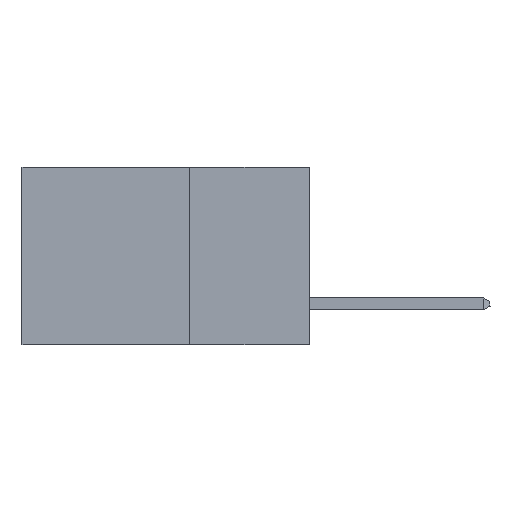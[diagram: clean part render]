
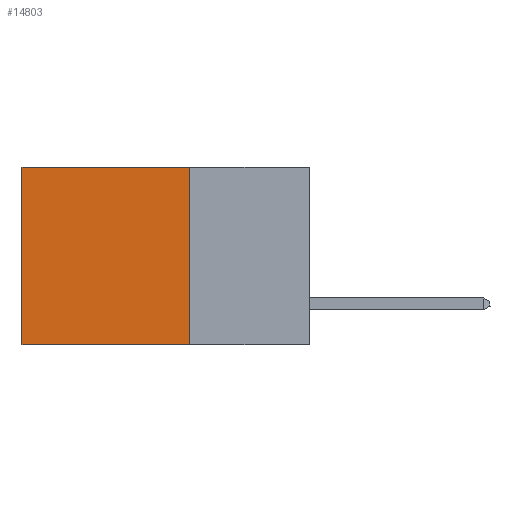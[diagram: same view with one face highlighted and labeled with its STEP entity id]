
A CAD part, left-side view. The second image highlights one B-rep face of the part: STEP entity #14803.
In plain terms, the highlighted planar face has unit normal (-1, 0, 0).
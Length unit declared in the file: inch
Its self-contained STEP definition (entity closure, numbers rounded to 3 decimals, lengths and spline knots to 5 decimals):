
#463 = LINE ( 'NONE', #3064, #1603 ) ;
#990 = EDGE_CURVE ( 'NONE', #2174, #29354, #23742, .T. ) ;
#1603 = VECTOR ( 'NONE', #5255, 39.37008 ) ;
#1618 = ORIENTED_EDGE ( 'NONE', *, *, #990, .F. ) ;
#2174 = VERTEX_POINT ( 'NONE', #26019 ) ;
#2418 = EDGE_CURVE ( 'NONE', #2174, #6714, #14458, .T. ) ;
#3064 = CARTESIAN_POINT ( 'NONE',  ( 0.2875, 0.6, 0. ) ) ;
#5183 = LINE ( 'NONE', #17685, #29901 ) ;
#5255 = DIRECTION ( 'NONE',  ( 0., 0., -1. ) ) ;
#6028 = CARTESIAN_POINT ( 'NONE',  ( 0.2875, 0.25, -0.37 ) ) ;
#6087 = CARTESIAN_POINT ( 'NONE',  ( 0.2875, 0.6, -0.37 ) ) ;
#6714 = VERTEX_POINT ( 'NONE', #15375 ) ;
#7618 = EDGE_LOOP ( 'NONE', ( #9112, #17664, #1618, #13158 ) ) ;
#9112 = ORIENTED_EDGE ( 'NONE', *, *, #25184, .T. ) ;
#12591 = DIRECTION ( 'NONE',  ( 0., 0., -1. ) ) ;
#13158 = ORIENTED_EDGE ( 'NONE', *, *, #2418, .T. ) ;
#13677 = VECTOR ( 'NONE', #21239, 39.37008 ) ;
#14458 = LINE ( 'NONE', #27015, #13677 ) ;
#14803 = ADVANCED_FACE ( 'NONE', ( #15764 ), #22045, .F. ) ;
#15057 = DIRECTION ( 'NONE',  ( 0., 1., 0. ) ) ;
#15375 = CARTESIAN_POINT ( 'NONE',  ( 0.2875, 0.6, 0. ) ) ;
#15764 = FACE_OUTER_BOUND ( 'NONE', #7618, .T. ) ;
#17251 = DIRECTION ( 'NONE',  ( 1., 0., 0. ) ) ;
#17372 = VECTOR ( 'NONE', #12591, 39.37008 ) ;
#17577 = AXIS2_PLACEMENT_3D ( 'NONE', #21949, #17251, #24589 ) ;
#17664 = ORIENTED_EDGE ( 'NONE', *, *, #19160, .F. ) ;
#17685 = CARTESIAN_POINT ( 'NONE',  ( 0.2875, 0.25, -0.37 ) ) ;
#19160 = EDGE_CURVE ( 'NONE', #29354, #25389, #5183, .T. ) ;
#19829 = CARTESIAN_POINT ( 'NONE',  ( 0.2875, 0.25, 0. ) ) ;
#21239 = DIRECTION ( 'NONE',  ( 0., 1., 0. ) ) ;
#21949 = CARTESIAN_POINT ( 'NONE',  ( 0.2875, 0.25, 0. ) ) ;
#22045 = PLANE ( 'NONE',  #17577 ) ;
#23742 = LINE ( 'NONE', #19829, #17372 ) ;
#24589 = DIRECTION ( 'NONE',  ( 0., 0., -1. ) ) ;
#25184 = EDGE_CURVE ( 'NONE', #6714, #25389, #463, .T. ) ;
#25389 = VERTEX_POINT ( 'NONE', #6087 ) ;
#26019 = CARTESIAN_POINT ( 'NONE',  ( 0.2875, 0.25, 0. ) ) ;
#27015 = CARTESIAN_POINT ( 'NONE',  ( 0.2875, 0.25, 0. ) ) ;
#29354 = VERTEX_POINT ( 'NONE', #6028 ) ;
#29901 = VECTOR ( 'NONE', #15057, 39.37008 ) ;
